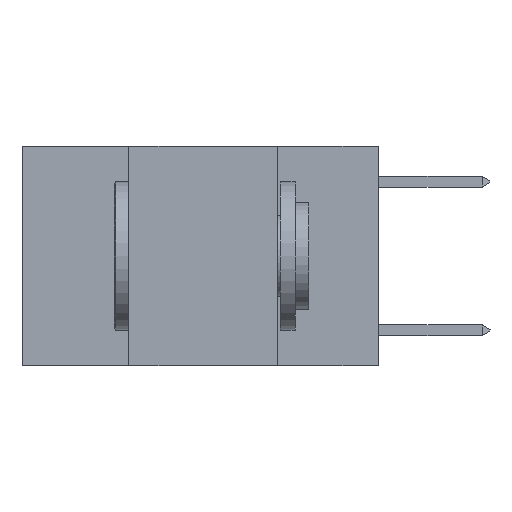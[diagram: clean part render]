
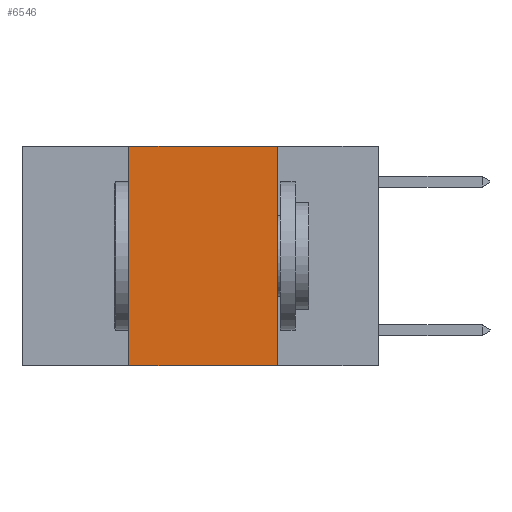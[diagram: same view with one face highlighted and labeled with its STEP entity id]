
A CAD part, left-side view. The second image highlights one B-rep face of the part: STEP entity #6546.
In plain terms, the highlighted planar face has unit normal (-1, 0, 0).
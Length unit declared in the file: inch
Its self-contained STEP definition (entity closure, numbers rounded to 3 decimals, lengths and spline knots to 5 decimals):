
#1320 = CARTESIAN_POINT ( 'NONE',  ( 0., 0.42, -0.37 ) ) ;
#1714 = EDGE_CURVE ( 'NONE', #15204, #9499, #24650, .T. ) ;
#1737 = VECTOR ( 'NONE', #11276, 39.37008 ) ;
#1821 = VECTOR ( 'NONE', #23553, 39.37008 ) ;
#1997 = DIRECTION ( 'NONE',  ( 1., 0., 0. ) ) ;
#3438 = VECTOR ( 'NONE', #14196, 39.37008 ) ;
#3961 = DIRECTION ( 'NONE',  ( 0., 0., -1. ) ) ;
#5790 = CARTESIAN_POINT ( 'NONE',  ( 0., 0.42, 0. ) ) ;
#6126 = EDGE_CURVE ( 'NONE', #15204, #23356, #18874, .T. ) ;
#6168 = FACE_OUTER_BOUND ( 'NONE', #19751, .T. ) ;
#6423 = AXIS2_PLACEMENT_3D ( 'NONE', #26556, #1997, #3961 ) ;
#6546 = ADVANCED_FACE ( 'NONE', ( #6168 ), #27076, .F. ) ;
#9499 = VERTEX_POINT ( 'NONE', #10853 ) ;
#9565 = ORIENTED_EDGE ( 'NONE', *, *, #22941, .F. ) ;
#10853 = CARTESIAN_POINT ( 'NONE',  ( 0., 0.42, 0. ) ) ;
#11276 = DIRECTION ( 'NONE',  ( 0., 0., -1. ) ) ;
#11398 = EDGE_CURVE ( 'NONE', #9499, #20005, #26204, .T. ) ;
#11637 = CARTESIAN_POINT ( 'NONE',  ( 0., 0.17, 0. ) ) ;
#14196 = DIRECTION ( 'NONE',  ( 0., 0., 1. ) ) ;
#14869 = VECTOR ( 'NONE', #15770, 39.37008 ) ;
#15204 = VERTEX_POINT ( 'NONE', #1320 ) ;
#15352 = ORIENTED_EDGE ( 'NONE', *, *, #11398, .F. ) ;
#15770 = DIRECTION ( 'NONE',  ( 0., -1., 0. ) ) ;
#17345 = LINE ( 'NONE', #21453, #1737 ) ;
#18874 = LINE ( 'NONE', #23139, #1821 ) ;
#19731 = CARTESIAN_POINT ( 'NONE',  ( 0., 0.6, 0. ) ) ;
#19751 = EDGE_LOOP ( 'NONE', ( #9565, #15352, #21471, #23996 ) ) ;
#20005 = VERTEX_POINT ( 'NONE', #11637 ) ;
#21453 = CARTESIAN_POINT ( 'NONE',  ( 0., 0.17, 0. ) ) ;
#21471 = ORIENTED_EDGE ( 'NONE', *, *, #1714, .F. ) ;
#22941 = EDGE_CURVE ( 'NONE', #20005, #23356, #17345, .T. ) ;
#23139 = CARTESIAN_POINT ( 'NONE',  ( 0., 0.6, -0.37 ) ) ;
#23356 = VERTEX_POINT ( 'NONE', #23357 ) ;
#23357 = CARTESIAN_POINT ( 'NONE',  ( 0., 0.17, -0.37 ) ) ;
#23553 = DIRECTION ( 'NONE',  ( 0., -1., 0. ) ) ;
#23996 = ORIENTED_EDGE ( 'NONE', *, *, #6126, .T. ) ;
#24650 = LINE ( 'NONE', #5790, #3438 ) ;
#26204 = LINE ( 'NONE', #19731, #14869 ) ;
#26556 = CARTESIAN_POINT ( 'NONE',  ( 0., 0.6, 0. ) ) ;
#27076 = PLANE ( 'NONE',  #6423 ) ;
